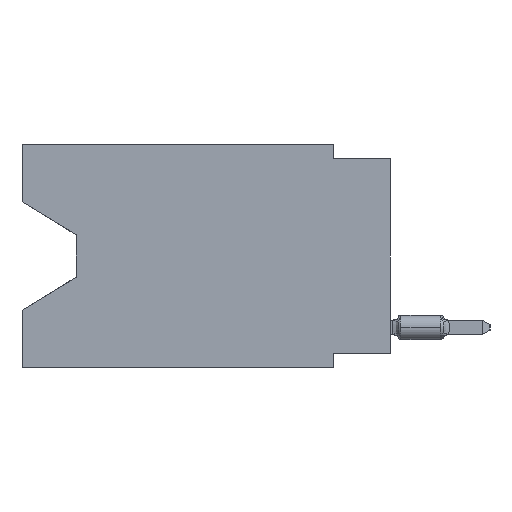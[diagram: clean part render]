
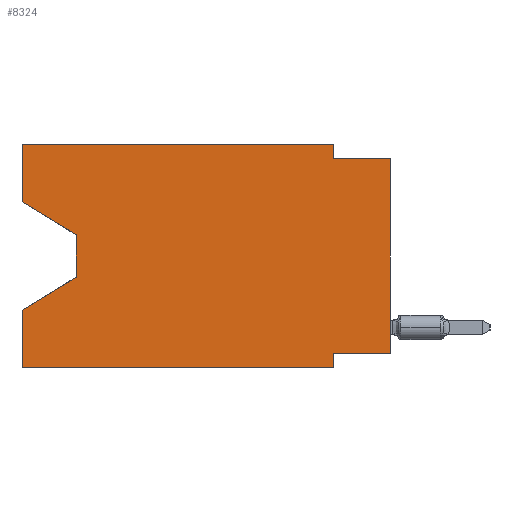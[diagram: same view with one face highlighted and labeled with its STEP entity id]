
A CAD part, left-side view. The second image highlights one B-rep face of the part: STEP entity #8324.
In plain terms, the highlighted planar face has unit normal (-1, 0, 0).
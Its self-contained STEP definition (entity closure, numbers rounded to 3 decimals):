
#186 = DIRECTION ( 'NONE',  ( 0., 0., -1. ) ) ;
#655 = EDGE_CURVE ( 'NONE', #45014, #77900, #81297, .T. ) ;
#1025 = LINE ( 'NONE', #27328, #81423 ) ;
#1057 = CARTESIAN_POINT ( 'NONE',  ( 0., 16.383, 0. ) ) ;
#1104 = VECTOR ( 'NONE', #10235, 1000. ) ;
#1652 = EDGE_CURVE ( 'NONE', #43189, #54266, #79990, .T. ) ;
#1730 = DIRECTION ( 'NONE',  ( 0., 0.855, -0.519 ) ) ;
#2520 = VERTEX_POINT ( 'NONE', #86918 ) ;
#2890 = CARTESIAN_POINT ( 'NONE',  ( 0., 0., -0.635 ) ) ;
#3286 = CARTESIAN_POINT ( 'NONE',  ( 0., 16.383, -9.906 ) ) ;
#8324 = ADVANCED_FACE ( 'NONE', ( #62118 ), #80854, .F. ) ;
#9412 = EDGE_CURVE ( 'NONE', #54266, #51519, #44481, .T. ) ;
#10235 = DIRECTION ( 'NONE',  ( 0., 0., -1. ) ) ;
#10496 = EDGE_CURVE ( 'NONE', #51519, #29847, #77470, .T. ) ;
#11352 = ORIENTED_EDGE ( 'NONE', *, *, #12159, .F. ) ;
#12071 = CARTESIAN_POINT ( 'NONE',  ( 0., 16.383, -9.906 ) ) ;
#12159 = EDGE_CURVE ( 'NONE', #77900, #2520, #57057, .T. ) ;
#15703 = VECTOR ( 'NONE', #50377, 1000. ) ;
#16228 = CARTESIAN_POINT ( 'NONE',  ( 0., 2.54, 0. ) ) ;
#17789 = VECTOR ( 'NONE', #56066, 1000. ) ;
#20496 = CARTESIAN_POINT ( 'NONE',  ( 0., 16.383, 0. ) ) ;
#21701 = VECTOR ( 'NONE', #47685, 1000. ) ;
#21713 = EDGE_CURVE ( 'NONE', #82774, #51695, #61908, .T. ) ;
#23180 = LINE ( 'NONE', #44562, #15703 ) ;
#26049 = ORIENTED_EDGE ( 'NONE', *, *, #31072, .T. ) ;
#27328 = CARTESIAN_POINT ( 'NONE',  ( 0., 16.383, 0. ) ) ;
#28239 = DIRECTION ( 'NONE',  ( 1., 0., 0. ) ) ;
#28866 = CARTESIAN_POINT ( 'NONE',  ( 0., 0., -0.635 ) ) ;
#29847 = VERTEX_POINT ( 'NONE', #55538 ) ;
#30450 = EDGE_CURVE ( 'NONE', #45014, #72737, #23180, .T. ) ;
#31072 = EDGE_CURVE ( 'NONE', #43182, #2520, #65139, .T. ) ;
#32521 = EDGE_CURVE ( 'NONE', #43182, #29847, #1025, .T. ) ;
#32754 = DIRECTION ( 'NONE',  ( 0., -0.855, -0.519 ) ) ;
#33470 = VECTOR ( 'NONE', #51176, 1000. ) ;
#36360 = CARTESIAN_POINT ( 'NONE',  ( 0., 16.383, 0. ) ) ;
#36987 = CARTESIAN_POINT ( 'NONE',  ( 0., 2.54, -9.906 ) ) ;
#37094 = VECTOR ( 'NONE', #32754, 1000. ) ;
#37582 = ORIENTED_EDGE ( 'NONE', *, *, #21713, .F. ) ;
#40501 = EDGE_CURVE ( 'NONE', #51695, #67940, #75530, .T. ) ;
#40605 = CARTESIAN_POINT ( 'NONE',  ( 0., 0., -9.271 ) ) ;
#42092 = AXIS2_PLACEMENT_3D ( 'NONE', #1057, #28239, #186 ) ;
#43182 = VERTEX_POINT ( 'NONE', #3286 ) ;
#43189 = VERTEX_POINT ( 'NONE', #78146 ) ;
#44481 = LINE ( 'NONE', #51611, #33470 ) ;
#44562 = CARTESIAN_POINT ( 'NONE',  ( 0., 0., 0. ) ) ;
#45014 = VERTEX_POINT ( 'NONE', #40605 ) ;
#47685 = DIRECTION ( 'NONE',  ( 0., 0., 1. ) ) ;
#47880 = EDGE_LOOP ( 'NONE', ( #59526, #58540, #61835, #82740, #26049, #11352, #62897, #51500, #75681, #72318, #37582, #69920 ) ) ;
#50377 = DIRECTION ( 'NONE',  ( 0., 0., 1. ) ) ;
#51176 = DIRECTION ( 'NONE',  ( 0., 0., -1. ) ) ;
#51500 = ORIENTED_EDGE ( 'NONE', *, *, #30450, .T. ) ;
#51519 = VERTEX_POINT ( 'NONE', #80023 ) ;
#51611 = CARTESIAN_POINT ( 'NONE',  ( 0., 13.97, -4.013 ) ) ;
#51695 = VERTEX_POINT ( 'NONE', #16228 ) ;
#51763 = DIRECTION ( 'NONE',  ( 0., -1., 0. ) ) ;
#53081 = CARTESIAN_POINT ( 'NONE',  ( 0., 2.54, -0.635 ) ) ;
#54266 = VERTEX_POINT ( 'NONE', #65798 ) ;
#54742 = CARTESIAN_POINT ( 'NONE',  ( 0., 16.383, 0. ) ) ;
#55051 = CARTESIAN_POINT ( 'NONE',  ( 0., 2.54, 0. ) ) ;
#55538 = CARTESIAN_POINT ( 'NONE',  ( 0., 16.383, -7.36 ) ) ;
#56066 = DIRECTION ( 'NONE',  ( 0., -1., 0. ) ) ;
#56350 = DIRECTION ( 'NONE',  ( 0., 0., -1. ) ) ;
#56873 = VECTOR ( 'NONE', #77776, 1000. ) ;
#57057 = LINE ( 'NONE', #36987, #1104 ) ;
#57489 = CARTESIAN_POINT ( 'NONE',  ( 0., 2.54, -9.271 ) ) ;
#58540 = ORIENTED_EDGE ( 'NONE', *, *, #9412, .T. ) ;
#59517 = CARTESIAN_POINT ( 'NONE',  ( 0., 16.383, -2.546 ) ) ;
#59526 = ORIENTED_EDGE ( 'NONE', *, *, #1652, .T. ) ;
#61835 = ORIENTED_EDGE ( 'NONE', *, *, #10496, .T. ) ;
#61908 = LINE ( 'NONE', #36360, #56873 ) ;
#62118 = FACE_OUTER_BOUND ( 'NONE', #47880, .T. ) ;
#62757 = LINE ( 'NONE', #28866, #17789 ) ;
#62897 = ORIENTED_EDGE ( 'NONE', *, *, #655, .F. ) ;
#65139 = LINE ( 'NONE', #12071, #85553 ) ;
#65798 = CARTESIAN_POINT ( 'NONE',  ( 0., 13.97, -4.013 ) ) ;
#66887 = EDGE_CURVE ( 'NONE', #43189, #82774, #81557, .T. ) ;
#67912 = DIRECTION ( 'NONE',  ( 0., 1., 0. ) ) ;
#67940 = VERTEX_POINT ( 'NONE', #53081 ) ;
#68865 = VECTOR ( 'NONE', #56350, 1000. ) ;
#69475 = CARTESIAN_POINT ( 'NONE',  ( 0., 13.97, -5.893 ) ) ;
#69920 = ORIENTED_EDGE ( 'NONE', *, *, #66887, .F. ) ;
#71643 = EDGE_CURVE ( 'NONE', #67940, #72737, #62757, .T. ) ;
#72318 = ORIENTED_EDGE ( 'NONE', *, *, #40501, .F. ) ;
#72737 = VERTEX_POINT ( 'NONE', #2890 ) ;
#75530 = LINE ( 'NONE', #55051, #68865 ) ;
#75681 = ORIENTED_EDGE ( 'NONE', *, *, #71643, .F. ) ;
#75925 = CARTESIAN_POINT ( 'NONE',  ( 0., 0., -9.271 ) ) ;
#77470 = LINE ( 'NONE', #69475, #87675 ) ;
#77776 = DIRECTION ( 'NONE',  ( 0., -1., 0. ) ) ;
#77900 = VERTEX_POINT ( 'NONE', #57489 ) ;
#78146 = CARTESIAN_POINT ( 'NONE',  ( 0., 16.383, -2.546 ) ) ;
#79990 = LINE ( 'NONE', #59517, #37094 ) ;
#80023 = CARTESIAN_POINT ( 'NONE',  ( 0., 13.97, -5.893 ) ) ;
#80854 = PLANE ( 'NONE',  #42092 ) ;
#81048 = VECTOR ( 'NONE', #67912, 1000. ) ;
#81297 = LINE ( 'NONE', #75925, #81048 ) ;
#81423 = VECTOR ( 'NONE', #83015, 1000. ) ;
#81557 = LINE ( 'NONE', #20496, #21701 ) ;
#82740 = ORIENTED_EDGE ( 'NONE', *, *, #32521, .F. ) ;
#82774 = VERTEX_POINT ( 'NONE', #54742 ) ;
#83015 = DIRECTION ( 'NONE',  ( 0., 0., 1. ) ) ;
#85553 = VECTOR ( 'NONE', #51763, 1000. ) ;
#86918 = CARTESIAN_POINT ( 'NONE',  ( 0., 2.54, -9.906 ) ) ;
#87675 = VECTOR ( 'NONE', #1730, 1000. ) ;
